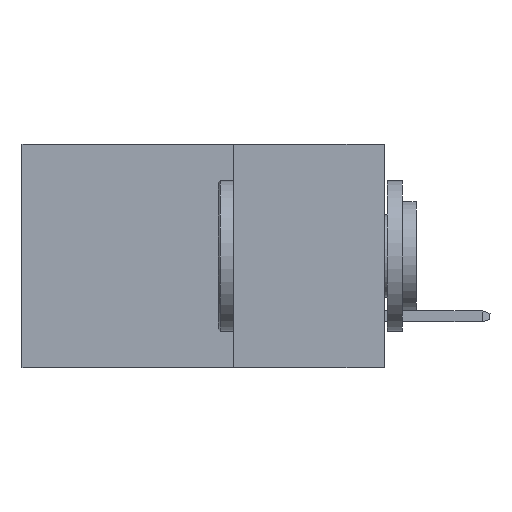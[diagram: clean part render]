
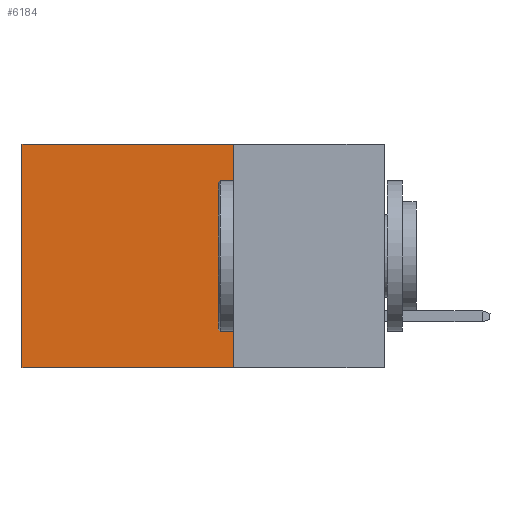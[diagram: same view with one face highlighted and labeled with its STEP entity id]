
A CAD part, left-side view. The second image highlights one B-rep face of the part: STEP entity #6184.
In plain terms, the highlighted planar face has unit normal (-1, 0, 0).
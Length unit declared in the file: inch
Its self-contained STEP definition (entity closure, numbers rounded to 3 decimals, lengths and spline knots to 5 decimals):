
#202 = ORIENTED_EDGE ( 'NONE', *, *, #1921, .T. ) ;
#292 = VERTEX_POINT ( 'NONE', #2473 ) ;
#368 = CARTESIAN_POINT ( 'NONE',  ( 0.2615, 0.25, 0. ) ) ;
#890 = EDGE_LOOP ( 'NONE', ( #202, #2629, #7486, #3779 ) ) ;
#1503 = LINE ( 'NONE', #8521, #6426 ) ;
#1532 = EDGE_CURVE ( 'NONE', #5657, #4565, #6089, .T. ) ;
#1830 = VECTOR ( 'NONE', #7383, 39.37008 ) ;
#1921 = EDGE_CURVE ( 'NONE', #4565, #292, #3613, .T. ) ;
#2473 = CARTESIAN_POINT ( 'NONE',  ( 0.2615, 0.6, -0.37 ) ) ;
#2594 = PLANE ( 'NONE',  #3908 ) ;
#2629 = ORIENTED_EDGE ( 'NONE', *, *, #8320, .F. ) ;
#2640 = FACE_OUTER_BOUND ( 'NONE', #890, .T. ) ;
#2992 = CARTESIAN_POINT ( 'NONE',  ( 0.2615, 0.25, -0.37 ) ) ;
#3019 = CARTESIAN_POINT ( 'NONE',  ( 0.2615, 0.6, -0.37 ) ) ;
#3613 = LINE ( 'NONE', #3019, #7693 ) ;
#3779 = ORIENTED_EDGE ( 'NONE', *, *, #1532, .T. ) ;
#3780 = VECTOR ( 'NONE', #6687, 39.37008 ) ;
#3908 = AXIS2_PLACEMENT_3D ( 'NONE', #4610, #8979, #5385 ) ;
#4291 = DIRECTION ( 'NONE',  ( 0., 0., -1. ) ) ;
#4565 = VERTEX_POINT ( 'NONE', #6808 ) ;
#4610 = CARTESIAN_POINT ( 'NONE',  ( 0.2615, 0.25, -0.37 ) ) ;
#5385 = DIRECTION ( 'NONE',  ( 0., 0., -1. ) ) ;
#5402 = LINE ( 'NONE', #6769, #3780 ) ;
#5657 = VERTEX_POINT ( 'NONE', #5903 ) ;
#5903 = CARTESIAN_POINT ( 'NONE',  ( 0.2615, 0.25, 0. ) ) ;
#6089 = LINE ( 'NONE', #368, #1830 ) ;
#6184 = ADVANCED_FACE ( 'NONE', ( #2640 ), #2594, .F. ) ;
#6412 = DIRECTION ( 'NONE',  ( 0., 0., -1. ) ) ;
#6426 = VECTOR ( 'NONE', #4291, 39.37008 ) ;
#6687 = DIRECTION ( 'NONE',  ( 0., 1., 0. ) ) ;
#6769 = CARTESIAN_POINT ( 'NONE',  ( 0.2615, 0.25, -0.37 ) ) ;
#6808 = CARTESIAN_POINT ( 'NONE',  ( 0.2615, 0.6, 0. ) ) ;
#7383 = DIRECTION ( 'NONE',  ( 0., 1., 0. ) ) ;
#7486 = ORIENTED_EDGE ( 'NONE', *, *, #8536, .F. ) ;
#7693 = VECTOR ( 'NONE', #6412, 39.37008 ) ;
#7781 = VERTEX_POINT ( 'NONE', #2992 ) ;
#8320 = EDGE_CURVE ( 'NONE', #7781, #292, #5402, .T. ) ;
#8521 = CARTESIAN_POINT ( 'NONE',  ( 0.2615, 0.25, -0.37 ) ) ;
#8536 = EDGE_CURVE ( 'NONE', #5657, #7781, #1503, .T. ) ;
#8979 = DIRECTION ( 'NONE',  ( 1., 0., 0. ) ) ;
